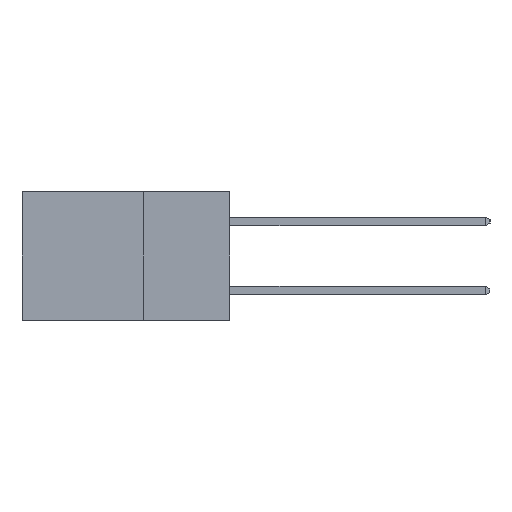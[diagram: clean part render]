
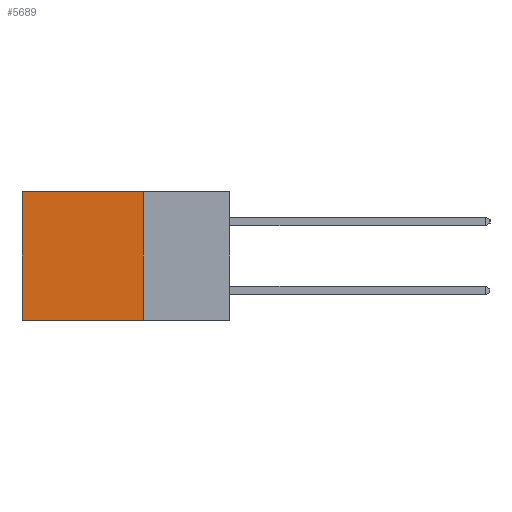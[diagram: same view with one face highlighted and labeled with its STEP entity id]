
A CAD part, left-side view. The second image highlights one B-rep face of the part: STEP entity #5689.
In plain terms, the highlighted planar face has unit normal (-1, 0, 0).
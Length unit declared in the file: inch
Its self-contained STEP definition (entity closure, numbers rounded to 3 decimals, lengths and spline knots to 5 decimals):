
#59 = FACE_OUTER_BOUND ( 'NONE', #12175, .T. ) ;
#175 = DIRECTION ( 'NONE',  ( 1., 0., 0. ) ) ;
#518 = DIRECTION ( 'NONE',  ( 0., 1., 0. ) ) ;
#548 = DIRECTION ( 'NONE',  ( 0., 0., -1. ) ) ;
#1176 = LINE ( 'NONE', #6844, #1467 ) ;
#1467 = VECTOR ( 'NONE', #6032, 39.37008 ) ;
#2426 = AXIS2_PLACEMENT_3D ( 'NONE', #3753, #175, #548 ) ;
#2889 = CARTESIAN_POINT ( 'NONE',  ( 0.298, 0.25, -0.37 ) ) ;
#3509 = EDGE_CURVE ( 'NONE', #8534, #4762, #1176, .T. ) ;
#3694 = CARTESIAN_POINT ( 'NONE',  ( 0.298, 0.25, -0.37 ) ) ;
#3753 = CARTESIAN_POINT ( 'NONE',  ( 0.298, 0.25, 0. ) ) ;
#3925 = CARTESIAN_POINT ( 'NONE',  ( 0.298, 0.6, 0. ) ) ;
#3979 = EDGE_CURVE ( 'NONE', #8534, #5537, #10322, .T. ) ;
#4762 = VERTEX_POINT ( 'NONE', #2889 ) ;
#5245 = VECTOR ( 'NONE', #518, 39.37008 ) ;
#5537 = VERTEX_POINT ( 'NONE', #3925 ) ;
#5689 = ADVANCED_FACE ( 'NONE', ( #59 ), #6099, .F. ) ;
#6032 = DIRECTION ( 'NONE',  ( 0., 0., -1. ) ) ;
#6099 = PLANE ( 'NONE',  #2426 ) ;
#6145 = CARTESIAN_POINT ( 'NONE',  ( 0.298, 0.6, -0.37 ) ) ;
#6307 = VERTEX_POINT ( 'NONE', #6145 ) ;
#6578 = ORIENTED_EDGE ( 'NONE', *, *, #11951, .T. ) ;
#6585 = LINE ( 'NONE', #10375, #8810 ) ;
#6619 = ORIENTED_EDGE ( 'NONE', *, *, #3979, .T. ) ;
#6844 = CARTESIAN_POINT ( 'NONE',  ( 0.298, 0.25, 0. ) ) ;
#7661 = EDGE_CURVE ( 'NONE', #4762, #6307, #11236, .T. ) ;
#8285 = VECTOR ( 'NONE', #12331, 39.37008 ) ;
#8396 = DIRECTION ( 'NONE',  ( 0., 0., -1. ) ) ;
#8534 = VERTEX_POINT ( 'NONE', #9694 ) ;
#8810 = VECTOR ( 'NONE', #8396, 39.37008 ) ;
#9264 = ORIENTED_EDGE ( 'NONE', *, *, #3509, .F. ) ;
#9694 = CARTESIAN_POINT ( 'NONE',  ( 0.298, 0.25, 0. ) ) ;
#10322 = LINE ( 'NONE', #12075, #5245 ) ;
#10375 = CARTESIAN_POINT ( 'NONE',  ( 0.298, 0.6, 0. ) ) ;
#11236 = LINE ( 'NONE', #3694, #8285 ) ;
#11420 = ORIENTED_EDGE ( 'NONE', *, *, #7661, .F. ) ;
#11951 = EDGE_CURVE ( 'NONE', #5537, #6307, #6585, .T. ) ;
#12075 = CARTESIAN_POINT ( 'NONE',  ( 0.298, 0.25, 0. ) ) ;
#12175 = EDGE_LOOP ( 'NONE', ( #6578, #11420, #9264, #6619 ) ) ;
#12331 = DIRECTION ( 'NONE',  ( 0., 1., 0. ) ) ;
